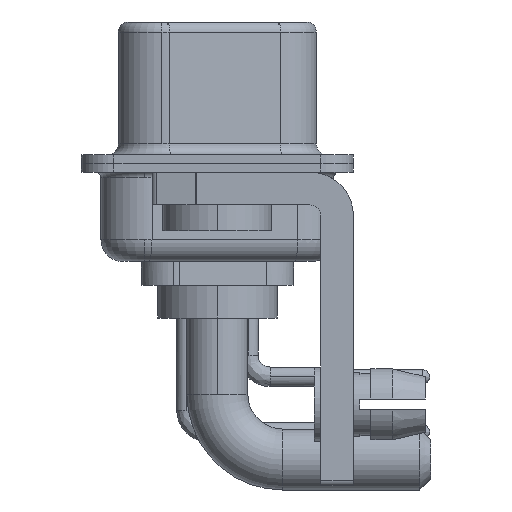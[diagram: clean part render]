
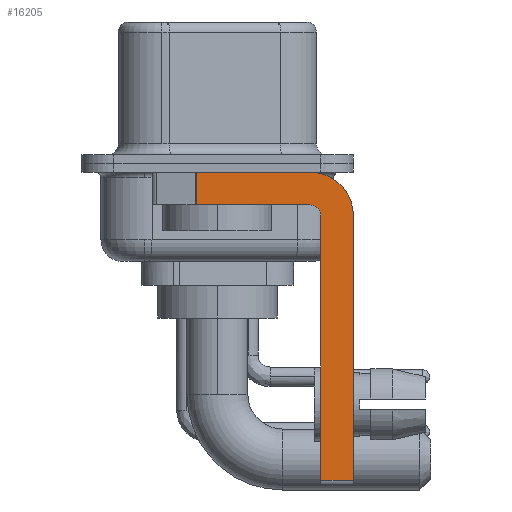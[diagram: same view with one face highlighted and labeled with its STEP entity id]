
A CAD part, left-side view. The second image highlights one B-rep face of the part: STEP entity #16205.
In plain terms, the highlighted planar face has unit normal (-1, 0, 0).
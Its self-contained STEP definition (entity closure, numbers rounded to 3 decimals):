
#475 = PLANE ( 'NONE',  #12347 ) ;
#930 = VERTEX_POINT ( 'NONE', #28515 ) ;
#1004 = CARTESIAN_POINT ( 'NONE',  ( -2.9, -6.25, -2.4 ) ) ;
#1064 = CARTESIAN_POINT ( 'NONE',  ( -2.9, 0.978, -0.4 ) ) ;
#1308 = DIRECTION ( 'NONE',  ( 0., 0., -1. ) ) ;
#1374 = LINE ( 'NONE', #15818, #23177 ) ;
#1985 = DIRECTION ( 'NONE',  ( 0., 0., -1. ) ) ;
#2592 = ORIENTED_EDGE ( 'NONE', *, *, #31029, .T. ) ;
#3132 = DIRECTION ( 'NONE',  ( 1., 0., 0. ) ) ;
#3683 = VERTEX_POINT ( 'NONE', #17454 ) ;
#4469 = EDGE_LOOP ( 'NONE', ( #5317, #2592, #25447, #18427, #12849, #22885, #24498, #26709 ) ) ;
#5132 = LINE ( 'NONE', #22277, #21660 ) ;
#5317 = ORIENTED_EDGE ( 'NONE', *, *, #5405, .F. ) ;
#5335 = VERTEX_POINT ( 'NONE', #1064 ) ;
#5405 = EDGE_CURVE ( 'NONE', #5335, #25938, #1374, .T. ) ;
#5912 = CIRCLE ( 'NONE', #7412, 0.5 ) ;
#5952 = CARTESIAN_POINT ( 'NONE',  ( -2.9, -4.25, -2.4 ) ) ;
#7410 = DIRECTION ( 'NONE',  ( 0., 0., -1. ) ) ;
#7412 = AXIS2_PLACEMENT_3D ( 'NONE', #10116, #7595, #24879 ) ;
#7595 = DIRECTION ( 'NONE',  ( -1., 0., 0. ) ) ;
#8285 = VERTEX_POINT ( 'NONE', #23966 ) ;
#9655 = VERTEX_POINT ( 'NONE', #15333 ) ;
#9713 = VERTEX_POINT ( 'NONE', #29981 ) ;
#10116 = CARTESIAN_POINT ( 'NONE',  ( -2.9, -4.25, -2.4 ) ) ;
#10537 = EDGE_CURVE ( 'NONE', #19845, #3683, #27507, .T. ) ;
#10594 = LINE ( 'NONE', #1004, #11885 ) ;
#11504 = LINE ( 'NONE', #14311, #27643 ) ;
#11885 = VECTOR ( 'NONE', #1308, 1000. ) ;
#12347 = AXIS2_PLACEMENT_3D ( 'NONE', #5952, #3132, #19962 ) ;
#12442 = DIRECTION ( 'NONE',  ( 1., 0., 0. ) ) ;
#12571 = FACE_OUTER_BOUND ( 'NONE', #4469, .T. ) ;
#12730 = CARTESIAN_POINT ( 'NONE',  ( -2.9, -4.75, -14.8 ) ) ;
#12849 = ORIENTED_EDGE ( 'NONE', *, *, #10537, .F. ) ;
#12945 = EDGE_CURVE ( 'NONE', #3683, #9713, #5912, .T. ) ;
#13185 = DIRECTION ( 'NONE',  ( 0., 0., 1. ) ) ;
#14311 = CARTESIAN_POINT ( 'NONE',  ( -2.9, -4.25, -1.9 ) ) ;
#14722 = DIRECTION ( 'NONE',  ( 0., -1., 0. ) ) ;
#15333 = CARTESIAN_POINT ( 'NONE',  ( -2.9, -6.25, -14.55 ) ) ;
#15818 = CARTESIAN_POINT ( 'NONE',  ( -2.9, 3., -0.4 ) ) ;
#16205 = ADVANCED_FACE ( 'NONE', ( #12571 ), #475, .F. ) ;
#16604 = EDGE_CURVE ( 'NONE', #25938, #930, #26916, .T. ) ;
#17454 = CARTESIAN_POINT ( 'NONE',  ( -2.9, -4.75, -2.4 ) ) ;
#18067 = VECTOR ( 'NONE', #1985, 1000. ) ;
#18427 = ORIENTED_EDGE ( 'NONE', *, *, #12945, .F. ) ;
#19845 = VERTEX_POINT ( 'NONE', #22047 ) ;
#19962 = DIRECTION ( 'NONE',  ( 0., 0., -1. ) ) ;
#20401 = DIRECTION ( 'NONE',  ( 0., -1., 0. ) ) ;
#20422 = VECTOR ( 'NONE', #13185, 1000. ) ;
#20851 = CARTESIAN_POINT ( 'NONE',  ( -2.9, 0.978, -1.9 ) ) ;
#21660 = VECTOR ( 'NONE', #14722, 1000. ) ;
#21838 = EDGE_CURVE ( 'NONE', #9713, #8285, #11504, .T. ) ;
#22047 = CARTESIAN_POINT ( 'NONE',  ( -2.9, -4.75, -14.55 ) ) ;
#22277 = CARTESIAN_POINT ( 'NONE',  ( -2.9, -4.25, -14.55 ) ) ;
#22885 = ORIENTED_EDGE ( 'NONE', *, *, #23272, .T. ) ;
#23177 = VECTOR ( 'NONE', #20401, 1000. ) ;
#23272 = EDGE_CURVE ( 'NONE', #19845, #9655, #5132, .T. ) ;
#23368 = LINE ( 'NONE', #20851, #18067 ) ;
#23422 = AXIS2_PLACEMENT_3D ( 'NONE', #28956, #12442, #7410 ) ;
#23912 = DIRECTION ( 'NONE',  ( 0., 1., 0. ) ) ;
#23966 = CARTESIAN_POINT ( 'NONE',  ( -2.9, 0.978, -1.9 ) ) ;
#24498 = ORIENTED_EDGE ( 'NONE', *, *, #27810, .F. ) ;
#24879 = DIRECTION ( 'NONE',  ( 0., 0., 1. ) ) ;
#24922 = CARTESIAN_POINT ( 'NONE',  ( -2.9, -4.25, -0.4 ) ) ;
#25447 = ORIENTED_EDGE ( 'NONE', *, *, #21838, .F. ) ;
#25938 = VERTEX_POINT ( 'NONE', #24922 ) ;
#26709 = ORIENTED_EDGE ( 'NONE', *, *, #16604, .F. ) ;
#26916 = CIRCLE ( 'NONE', #23422, 2. ) ;
#27507 = LINE ( 'NONE', #12730, #20422 ) ;
#27643 = VECTOR ( 'NONE', #23912, 1000. ) ;
#27810 = EDGE_CURVE ( 'NONE', #930, #9655, #10594, .T. ) ;
#28515 = CARTESIAN_POINT ( 'NONE',  ( -2.9, -6.25, -2.4 ) ) ;
#28956 = CARTESIAN_POINT ( 'NONE',  ( -2.9, -4.25, -2.4 ) ) ;
#29981 = CARTESIAN_POINT ( 'NONE',  ( -2.9, -4.25, -1.9 ) ) ;
#31029 = EDGE_CURVE ( 'NONE', #5335, #8285, #23368, .T. ) ;
